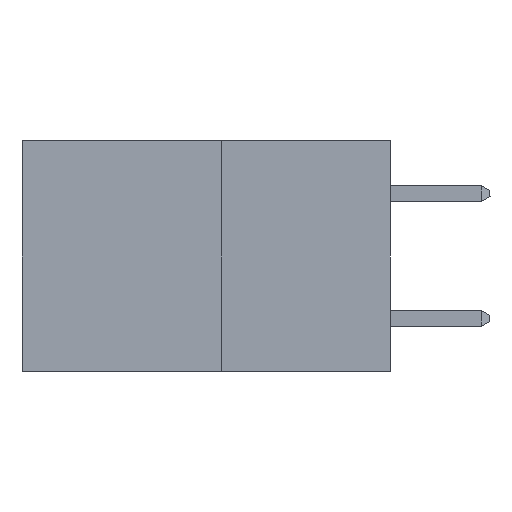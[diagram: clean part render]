
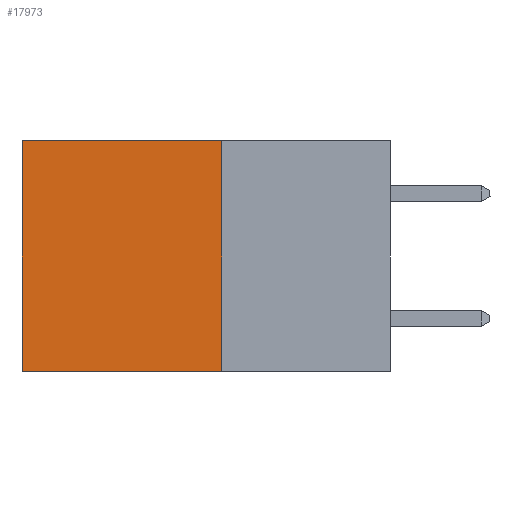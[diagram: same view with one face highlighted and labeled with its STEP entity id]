
A CAD part, left-side view. The second image highlights one B-rep face of the part: STEP entity #17973.
In plain terms, the highlighted planar face has unit normal (-1, 0, 0).
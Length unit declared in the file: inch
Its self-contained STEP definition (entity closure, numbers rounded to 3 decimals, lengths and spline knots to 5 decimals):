
#1674 = CARTESIAN_POINT ( 'NONE',  ( 0.277, 0.27, -0.37 ) ) ;
#2933 = EDGE_CURVE ( 'NONE', #18520, #20331, #17355, .T. ) ;
#2966 = EDGE_LOOP ( 'NONE', ( #11499, #6546, #7893, #14162 ) ) ;
#2980 = CARTESIAN_POINT ( 'NONE',  ( 0.277, 0.27, -0.37 ) ) ;
#3772 = VERTEX_POINT ( 'NONE', #8558 ) ;
#4062 = FACE_OUTER_BOUND ( 'NONE', #2966, .T. ) ;
#4068 = CARTESIAN_POINT ( 'NONE',  ( 0.277, 0.27, 0. ) ) ;
#5516 = DIRECTION ( 'NONE',  ( 1., 0., 0. ) ) ;
#5702 = EDGE_CURVE ( 'NONE', #26629, #20331, #7999, .T. ) ;
#6190 = DIRECTION ( 'NONE',  ( 0., 1., 0. ) ) ;
#6546 = ORIENTED_EDGE ( 'NONE', *, *, #2933, .F. ) ;
#7325 = VECTOR ( 'NONE', #15617, 39.37008 ) ;
#7893 = ORIENTED_EDGE ( 'NONE', *, *, #15752, .F. ) ;
#7999 = LINE ( 'NONE', #15920, #7325 ) ;
#8558 = CARTESIAN_POINT ( 'NONE',  ( 0.277, 0.27, 0. ) ) ;
#10671 = CARTESIAN_POINT ( 'NONE',  ( 0.277, 0.59, -0.37 ) ) ;
#11499 = ORIENTED_EDGE ( 'NONE', *, *, #5702, .T. ) ;
#12398 = VECTOR ( 'NONE', #24991, 39.37008 ) ;
#12468 = VECTOR ( 'NONE', #6190, 39.37008 ) ;
#13144 = LINE ( 'NONE', #4068, #12468 ) ;
#13823 = PLANE ( 'NONE',  #18858 ) ;
#14162 = ORIENTED_EDGE ( 'NONE', *, *, #14876, .T. ) ;
#14876 = EDGE_CURVE ( 'NONE', #3772, #26629, #13144, .T. ) ;
#15617 = DIRECTION ( 'NONE',  ( 0., 0., -1. ) ) ;
#15752 = EDGE_CURVE ( 'NONE', #3772, #18520, #19365, .T. ) ;
#15920 = CARTESIAN_POINT ( 'NONE',  ( 0.277, 0.59, -0.37 ) ) ;
#17355 = LINE ( 'NONE', #1674, #12398 ) ;
#17668 = CARTESIAN_POINT ( 'NONE',  ( 0.277, 0.27, -0.37 ) ) ;
#17973 = ADVANCED_FACE ( 'NONE', ( #4062 ), #13823, .F. ) ;
#18174 = CARTESIAN_POINT ( 'NONE',  ( 0.277, 0.27, -0.37 ) ) ;
#18520 = VERTEX_POINT ( 'NONE', #17668 ) ;
#18858 = AXIS2_PLACEMENT_3D ( 'NONE', #18174, #5516, #20300 ) ;
#19365 = LINE ( 'NONE', #2980, #24429 ) ;
#20300 = DIRECTION ( 'NONE',  ( 0., 0., -1. ) ) ;
#20331 = VERTEX_POINT ( 'NONE', #10671 ) ;
#21625 = DIRECTION ( 'NONE',  ( 0., 0., -1. ) ) ;
#24429 = VECTOR ( 'NONE', #21625, 39.37008 ) ;
#24991 = DIRECTION ( 'NONE',  ( 0., 1., 0. ) ) ;
#26629 = VERTEX_POINT ( 'NONE', #27148 ) ;
#27148 = CARTESIAN_POINT ( 'NONE',  ( 0.277, 0.59, 0. ) ) ;
